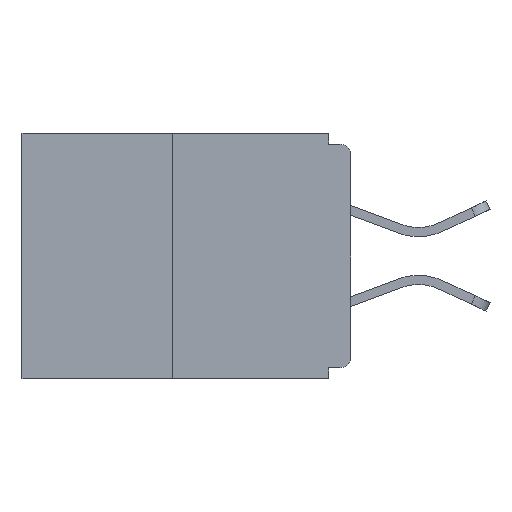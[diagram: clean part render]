
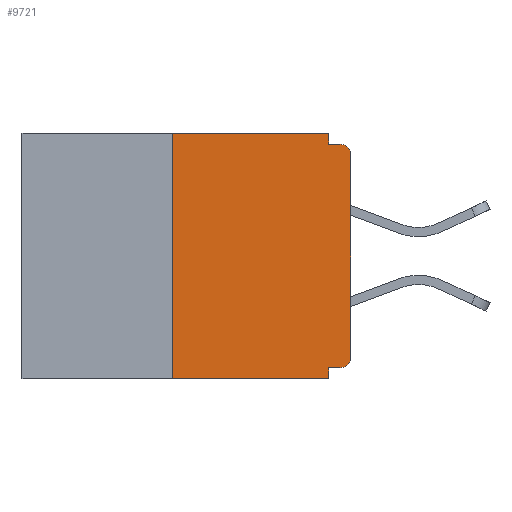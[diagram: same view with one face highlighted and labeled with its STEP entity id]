
A CAD part, left-side view. The second image highlights one B-rep face of the part: STEP entity #9721.
In plain terms, the highlighted planar face has unit normal (-1, 0, 0).
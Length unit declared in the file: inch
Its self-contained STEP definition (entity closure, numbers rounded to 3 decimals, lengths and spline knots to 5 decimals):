
#59 = EDGE_CURVE ( 'NONE', #6616, #12524, #16233, .T. ) ;
#105 = EDGE_CURVE ( 'NONE', #15493, #11065, #4623, .T. ) ;
#417 = ORIENTED_EDGE ( 'NONE', *, *, #3297, .F. ) ;
#722 = CARTESIAN_POINT ( 'NONE',  ( 0., 0.25, -0.343 ) ) ;
#780 = LINE ( 'NONE', #10914, #5013 ) ;
#828 = VECTOR ( 'NONE', #12657, 39.37008 ) ;
#860 = AXIS2_PLACEMENT_3D ( 'NONE', #3577, #14848, #6869 ) ;
#2330 = CARTESIAN_POINT ( 'NONE',  ( 0., 0.015, -0.328 ) ) ;
#2597 = LINE ( 'NONE', #4046, #6879 ) ;
#2677 = VERTEX_POINT ( 'NONE', #11382 ) ;
#3297 = EDGE_CURVE ( 'NONE', #11581, #6616, #3530, .T. ) ;
#3530 = LINE ( 'NONE', #16368, #9540 ) ;
#3577 = CARTESIAN_POINT ( 'NONE',  ( 0., 0.46, 0. ) ) ;
#3668 = DIRECTION ( 'NONE',  ( 0., 0., -1. ) ) ;
#4025 = CARTESIAN_POINT ( 'NONE',  ( 0., 0.015, -0.015 ) ) ;
#4046 = CARTESIAN_POINT ( 'NONE',  ( 0., 0.46, 0. ) ) ;
#4623 = CIRCLE ( 'NONE', #16606, 0.015 ) ;
#4962 = VERTEX_POINT ( 'NONE', #722 ) ;
#5013 = VECTOR ( 'NONE', #17307, 39.37008 ) ;
#5049 = EDGE_CURVE ( 'NONE', #2677, #15493, #18111, .T. ) ;
#6069 = ORIENTED_EDGE ( 'NONE', *, *, #59, .F. ) ;
#6074 = DIRECTION ( 'NONE',  ( 0., 0., -1. ) ) ;
#6251 = DIRECTION ( 'NONE',  ( 0., 0., 1. ) ) ;
#6616 = VERTEX_POINT ( 'NONE', #19839 ) ;
#6679 = DIRECTION ( 'NONE',  ( 0., 0., -1. ) ) ;
#6869 = DIRECTION ( 'NONE',  ( 0., 0., -1. ) ) ;
#6879 = VECTOR ( 'NONE', #20213, 39.37008 ) ;
#7799 = CARTESIAN_POINT ( 'NONE',  ( 0., 0.46, -0.343 ) ) ;
#8262 = EDGE_CURVE ( 'NONE', #4962, #12524, #15445, .T. ) ;
#8312 = ORIENTED_EDGE ( 'NONE', *, *, #13305, .F. ) ;
#8338 = CARTESIAN_POINT ( 'NONE',  ( 0., 0.031, -0.015 ) ) ;
#8385 = CARTESIAN_POINT ( 'NONE',  ( 0., 0.25, 0. ) ) ;
#8829 = CARTESIAN_POINT ( 'NONE',  ( 0., 0.031, -0.343 ) ) ;
#9003 = VERTEX_POINT ( 'NONE', #13569 ) ;
#9096 = VECTOR ( 'NONE', #17506, 39.37008 ) ;
#9144 = CARTESIAN_POINT ( 'NONE',  ( 0., 0., -0.03 ) ) ;
#9169 = DIRECTION ( 'NONE',  ( -1., 0., 0. ) ) ;
#9211 = VERTEX_POINT ( 'NONE', #8385 ) ;
#9540 = VECTOR ( 'NONE', #13354, 39.37008 ) ;
#9721 = ADVANCED_FACE ( 'NONE', ( #19834 ), #17900, .F. ) ;
#9884 = EDGE_CURVE ( 'NONE', #4962, #9211, #780, .T. ) ;
#10914 = CARTESIAN_POINT ( 'NONE',  ( 0., 0.25, 0. ) ) ;
#10969 = EDGE_CURVE ( 'NONE', #11581, #2677, #13066, .T. ) ;
#11038 = CARTESIAN_POINT ( 'NONE',  ( 0., 0., 0. ) ) ;
#11054 = EDGE_LOOP ( 'NONE', ( #14545, #16367, #20266, #6069, #417, #13076, #14843, #13081, #12118, #8312 ) ) ;
#11065 = VERTEX_POINT ( 'NONE', #4025 ) ;
#11382 = CARTESIAN_POINT ( 'NONE',  ( 0., 0., -0.313 ) ) ;
#11581 = VERTEX_POINT ( 'NONE', #2330 ) ;
#11991 = VECTOR ( 'NONE', #6251, 39.37008 ) ;
#12118 = ORIENTED_EDGE ( 'NONE', *, *, #18953, .F. ) ;
#12524 = VERTEX_POINT ( 'NONE', #14611 ) ;
#12526 = VERTEX_POINT ( 'NONE', #8338 ) ;
#12657 = DIRECTION ( 'NONE',  ( 0., -1., 0. ) ) ;
#12702 = CARTESIAN_POINT ( 'NONE',  ( 0., 0.015, -0.03 ) ) ;
#12969 = VECTOR ( 'NONE', #6679, 39.37008 ) ;
#13066 = CIRCLE ( 'NONE', #18051, 0.015 ) ;
#13076 = ORIENTED_EDGE ( 'NONE', *, *, #10969, .T. ) ;
#13081 = ORIENTED_EDGE ( 'NONE', *, *, #105, .T. ) ;
#13305 = EDGE_CURVE ( 'NONE', #9003, #12526, #16507, .T. ) ;
#13324 = DIRECTION ( 'NONE',  ( -1., 0., 0. ) ) ;
#13354 = DIRECTION ( 'NONE',  ( 0., 1., 0. ) ) ;
#13569 = CARTESIAN_POINT ( 'NONE',  ( 0., 0.031, 0. ) ) ;
#14096 = CARTESIAN_POINT ( 'NONE',  ( 0., 0., -0.015 ) ) ;
#14545 = ORIENTED_EDGE ( 'NONE', *, *, #18912, .F. ) ;
#14611 = CARTESIAN_POINT ( 'NONE',  ( 0., 0.031, -0.343 ) ) ;
#14843 = ORIENTED_EDGE ( 'NONE', *, *, #5049, .T. ) ;
#14848 = DIRECTION ( 'NONE',  ( 1., 0., 0. ) ) ;
#14970 = LINE ( 'NONE', #14096, #9096 ) ;
#15445 = LINE ( 'NONE', #7799, #828 ) ;
#15493 = VERTEX_POINT ( 'NONE', #9144 ) ;
#16233 = LINE ( 'NONE', #8829, #20580 ) ;
#16367 = ORIENTED_EDGE ( 'NONE', *, *, #9884, .F. ) ;
#16368 = CARTESIAN_POINT ( 'NONE',  ( 0., 0., -0.328 ) ) ;
#16507 = LINE ( 'NONE', #17856, #12969 ) ;
#16606 = AXIS2_PLACEMENT_3D ( 'NONE', #12702, #9169, #6074 ) ;
#17307 = DIRECTION ( 'NONE',  ( 0., 0., 1. ) ) ;
#17506 = DIRECTION ( 'NONE',  ( 0., -1., 0. ) ) ;
#17856 = CARTESIAN_POINT ( 'NONE',  ( 0., 0.031, 0. ) ) ;
#17900 = PLANE ( 'NONE',  #860 ) ;
#18051 = AXIS2_PLACEMENT_3D ( 'NONE', #19784, #13324, #3668 ) ;
#18111 = LINE ( 'NONE', #11038, #11991 ) ;
#18912 = EDGE_CURVE ( 'NONE', #9211, #9003, #2597, .T. ) ;
#18953 = EDGE_CURVE ( 'NONE', #12526, #11065, #14970, .T. ) ;
#19784 = CARTESIAN_POINT ( 'NONE',  ( 0., 0.015, -0.313 ) ) ;
#19834 = FACE_OUTER_BOUND ( 'NONE', #11054, .T. ) ;
#19839 = CARTESIAN_POINT ( 'NONE',  ( 0., 0.031, -0.328 ) ) ;
#20213 = DIRECTION ( 'NONE',  ( 0., -1., 0. ) ) ;
#20266 = ORIENTED_EDGE ( 'NONE', *, *, #8262, .T. ) ;
#20390 = DIRECTION ( 'NONE',  ( 0., 0., -1. ) ) ;
#20580 = VECTOR ( 'NONE', #20390, 39.37008 ) ;
